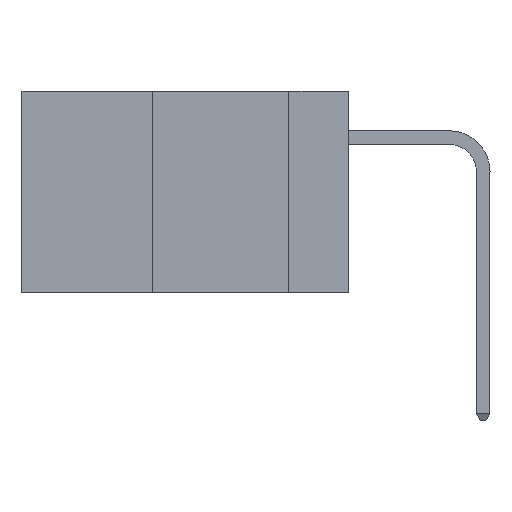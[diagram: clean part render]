
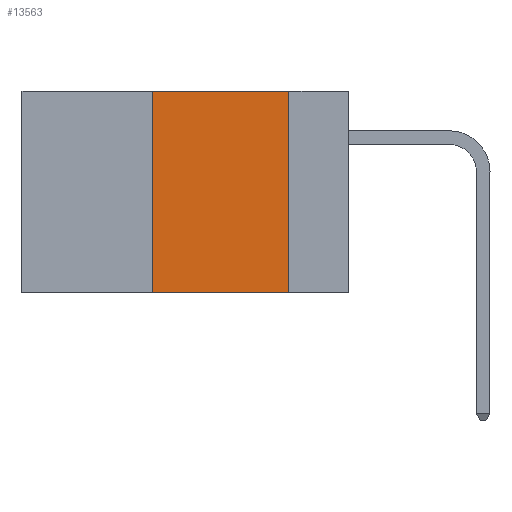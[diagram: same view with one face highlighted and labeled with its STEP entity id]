
A CAD part, left-side view. The second image highlights one B-rep face of the part: STEP entity #13563.
In plain terms, the highlighted planar face has unit normal (-1, 0, 0).
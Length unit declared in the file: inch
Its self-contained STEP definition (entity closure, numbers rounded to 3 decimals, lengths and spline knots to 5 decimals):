
#2386 = AXIS2_PLACEMENT_3D ( 'NONE', #6809, #24748, #9379 ) ;
#3842 = VERTEX_POINT ( 'NONE', #25458 ) ;
#4143 = CARTESIAN_POINT ( 'NONE',  ( 0., 0.6, -0.37 ) ) ;
#5668 = CARTESIAN_POINT ( 'NONE',  ( 0., 0.11, 0. ) ) ;
#5704 = EDGE_CURVE ( 'NONE', #26259, #29760, #17955, .T. ) ;
#6809 = CARTESIAN_POINT ( 'NONE',  ( 0., 0.6, 0. ) ) ;
#7194 = VECTOR ( 'NONE', #25253, 39.37008 ) ;
#7395 = CARTESIAN_POINT ( 'NONE',  ( 0., 0.11, -0.37 ) ) ;
#7777 = EDGE_LOOP ( 'NONE', ( #10121, #24116, #12076, #29336 ) ) ;
#8058 = DIRECTION ( 'NONE',  ( 0., 0., -1. ) ) ;
#9379 = DIRECTION ( 'NONE',  ( 0., 0., -1. ) ) ;
#10121 = ORIENTED_EDGE ( 'NONE', *, *, #23925, .F. ) ;
#10214 = LINE ( 'NONE', #5668, #29810 ) ;
#12076 = ORIENTED_EDGE ( 'NONE', *, *, #5704, .F. ) ;
#12343 = EDGE_CURVE ( 'NONE', #29760, #3842, #14076, .T. ) ;
#13563 = ADVANCED_FACE ( 'NONE', ( #23183 ), #19639, .F. ) ;
#14076 = LINE ( 'NONE', #22716, #7194 ) ;
#14916 = VERTEX_POINT ( 'NONE', #7395 ) ;
#16109 = VECTOR ( 'NONE', #22098, 39.37008 ) ;
#17170 = VECTOR ( 'NONE', #28011, 39.37008 ) ;
#17955 = LINE ( 'NONE', #25465, #17170 ) ;
#19639 = PLANE ( 'NONE',  #2386 ) ;
#22098 = DIRECTION ( 'NONE',  ( 0., -1., 0. ) ) ;
#22639 = CARTESIAN_POINT ( 'NONE',  ( 0., 0.36, 0. ) ) ;
#22716 = CARTESIAN_POINT ( 'NONE',  ( 0., 0.6, 0. ) ) ;
#22980 = CARTESIAN_POINT ( 'NONE',  ( 0., 0.36, -0.37 ) ) ;
#23183 = FACE_OUTER_BOUND ( 'NONE', #7777, .T. ) ;
#23925 = EDGE_CURVE ( 'NONE', #3842, #14916, #10214, .T. ) ;
#24116 = ORIENTED_EDGE ( 'NONE', *, *, #12343, .F. ) ;
#24748 = DIRECTION ( 'NONE',  ( 1., 0., 0. ) ) ;
#25253 = DIRECTION ( 'NONE',  ( 0., -1., 0. ) ) ;
#25458 = CARTESIAN_POINT ( 'NONE',  ( 0., 0.11, 0. ) ) ;
#25465 = CARTESIAN_POINT ( 'NONE',  ( 0., 0.36, 0. ) ) ;
#26019 = EDGE_CURVE ( 'NONE', #26259, #14916, #29660, .T. ) ;
#26259 = VERTEX_POINT ( 'NONE', #22980 ) ;
#28011 = DIRECTION ( 'NONE',  ( 0., 0., 1. ) ) ;
#29336 = ORIENTED_EDGE ( 'NONE', *, *, #26019, .T. ) ;
#29660 = LINE ( 'NONE', #4143, #16109 ) ;
#29760 = VERTEX_POINT ( 'NONE', #22639 ) ;
#29810 = VECTOR ( 'NONE', #8058, 39.37008 ) ;
